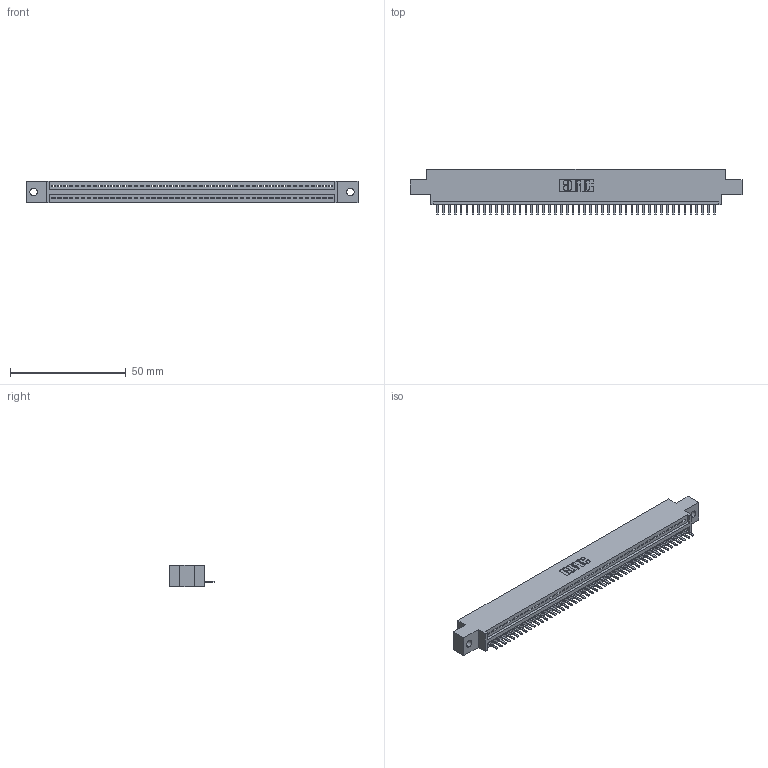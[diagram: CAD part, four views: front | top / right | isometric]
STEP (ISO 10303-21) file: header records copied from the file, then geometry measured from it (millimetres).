
FILE_DESCRIPTION (( 'STEP AP203' ), '1' );
FILE_NAME ('345-048-520-602.STEP', '2019-10-09T04:13:15', ( '' ), ( '' ), 'SwSTEP 2.0', 'SolidWorks 2016', '' );
FILE_SCHEMA (( 'CONFIG_CONTROL_DESIGN' ));
Length unit declared in the file: inch
Products named in the file (3): 345-048-520-602; 345 Part_0.170 Offset - 0.128 Dia; 345-292-001_345-293-120
Assembly tree (49 placements, depth 2):
  345-048-520-602
    345 Part_0.170 Offset - 0.128 Dia
    345-292-001_345-293-120  x48
Bounding box: 143.13 x 19.68 x 9.4 mm (x, y, z)
Volume: 13355.5 mm3; surface area: 17233.2 mm2
Topology: 49 solids, 49 shells, 3106 faces, 9185 edges, 5994 vertices
Faces by surface type: plane 2100, cylinder 1006
Entity records: 35567 total; most frequent: CARTESIAN_POINT 6180, ORIENTED_EDGE 6150, DIRECTION 5375, EDGE_CURVE 3075, VECTOR 2747, LINE 2747, VERTEX_POINT 2046, AXIS2_PLACEMENT_3D 1314
